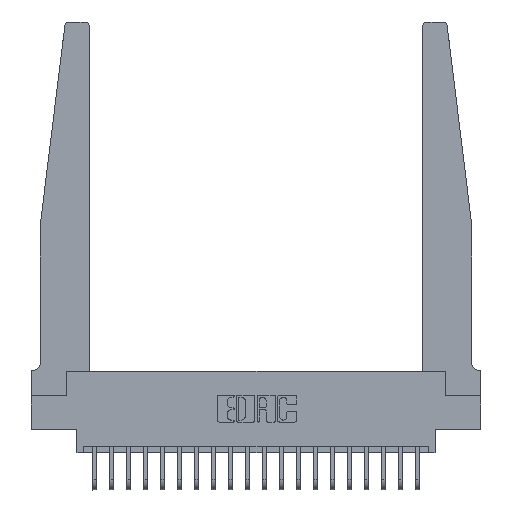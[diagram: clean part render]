
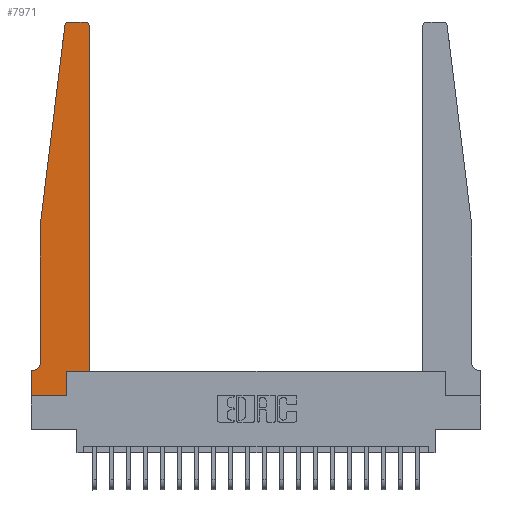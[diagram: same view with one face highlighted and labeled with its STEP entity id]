
A CAD part, top view. The second image highlights one B-rep face of the part: STEP entity #7971.
In plain terms, the highlighted planar face has unit normal (0, 0, 1).
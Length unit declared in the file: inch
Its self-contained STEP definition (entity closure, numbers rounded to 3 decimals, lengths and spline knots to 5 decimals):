
#485 = CARTESIAN_POINT ( 'NONE',  ( 0.015, 0.2375, 0.37 ) ) ;
#555 = VECTOR ( 'NONE', #1249, 39.37008 ) ;
#657 = DIRECTION ( 'NONE',  ( 1., 0., 0. ) ) ;
#1044 = CARTESIAN_POINT ( 'NONE',  ( 0.065, 1.25, 0.37 ) ) ;
#1048 = ORIENTED_EDGE ( 'NONE', *, *, #9518, .T. ) ;
#1143 = DIRECTION ( 'NONE',  ( 1., 0., 0. ) ) ;
#1249 = DIRECTION ( 'NONE',  ( 0., -1., 0. ) ) ;
#1559 = CIRCLE ( 'NONE', #14652, 0.03 ) ;
#1574 = CARTESIAN_POINT ( 'NONE',  ( 0.25, 2.75, 0.37 ) ) ;
#1659 = EDGE_CURVE ( 'NONE', #12723, #5210, #11822, .T. ) ;
#1767 = DIRECTION ( 'NONE',  ( 1., 0., 0. ) ) ;
#1916 = LINE ( 'NONE', #14757, #15223 ) ;
#2643 = ORIENTED_EDGE ( 'NONE', *, *, #12371, .T. ) ;
#2938 = DIRECTION ( 'NONE',  ( 0., 1., 0. ) ) ;
#3005 = CARTESIAN_POINT ( 'NONE',  ( 0., 0.1875, 0.37 ) ) ;
#3436 = ORIENTED_EDGE ( 'NONE', *, *, #12377, .T. ) ;
#3744 = DIRECTION ( 'NONE',  ( -1., 0., 0. ) ) ;
#4289 = VERTEX_POINT ( 'NONE', #7730 ) ;
#4322 = EDGE_CURVE ( 'NONE', #10886, #17482, #1916, .T. ) ;
#4595 = ORIENTED_EDGE ( 'NONE', *, *, #11111, .T. ) ;
#4912 = EDGE_CURVE ( 'NONE', #7193, #10886, #7055, .T. ) ;
#4939 = CARTESIAN_POINT ( 'NONE',  ( 0.065, 1.25, 0.37 ) ) ;
#5179 = VERTEX_POINT ( 'NONE', #4939 ) ;
#5210 = VERTEX_POINT ( 'NONE', #9680 ) ;
#5253 = AXIS2_PLACEMENT_3D ( 'NONE', #9687, #16196, #1767 ) ;
#5894 = DIRECTION ( 'NONE',  ( -0.122, -0.992, 0. ) ) ;
#6666 = ORIENTED_EDGE ( 'NONE', *, *, #4322, .T. ) ;
#7055 = LINE ( 'NONE', #13475, #9203 ) ;
#7065 = EDGE_LOOP ( 'NONE', ( #2643, #1048, #4595, #18231, #11783, #8671, #16813, #6666, #3436, #19146, #17581, #16800 ) ) ;
#7193 = VERTEX_POINT ( 'NONE', #3005 ) ;
#7730 = CARTESIAN_POINT ( 'NONE',  ( 0.24675, 2.72367, 0.37 ) ) ;
#7766 = CARTESIAN_POINT ( 'NONE',  ( 0.2605, 0.18, 0.37 ) ) ;
#7785 = FACE_OUTER_BOUND ( 'NONE', #7065, .T. ) ;
#7890 = LINE ( 'NONE', #1574, #15071 ) ;
#7891 = PLANE ( 'NONE',  #5253 ) ;
#7971 = ADVANCED_FACE ( 'NONE', ( #7785 ), #7891, .T. ) ;
#8057 = AXIS2_PLACEMENT_3D ( 'NONE', #485, #19723, #3744 ) ;
#8364 = CARTESIAN_POINT ( 'NONE',  ( 0.015, 0.1875, 0.37 ) ) ;
#8671 = ORIENTED_EDGE ( 'NONE', *, *, #13625, .T. ) ;
#8812 = CARTESIAN_POINT ( 'NONE',  ( 0.395, 2.75, 0.37 ) ) ;
#8916 = EDGE_CURVE ( 'NONE', #5210, #16633, #20361, .T. ) ;
#9148 = CARTESIAN_POINT ( 'NONE',  ( 0.27653, 2.72, 0.37 ) ) ;
#9203 = VECTOR ( 'NONE', #19871, 39.37008 ) ;
#9220 = CARTESIAN_POINT ( 'NONE',  ( 0.395, 2.72, 0.37 ) ) ;
#9425 = EDGE_CURVE ( 'NONE', #5179, #15299, #15664, .T. ) ;
#9518 = EDGE_CURVE ( 'NONE', #15981, #4289, #1559, .T. ) ;
#9571 = VERTEX_POINT ( 'NONE', #7766 ) ;
#9680 = CARTESIAN_POINT ( 'NONE',  ( 0.425, 2.72, 0.37 ) ) ;
#9687 = CARTESIAN_POINT ( 'NONE',  ( 0., 0.1875, 0.37 ) ) ;
#10753 = VECTOR ( 'NONE', #15056, 39.37008 ) ;
#10886 = VERTEX_POINT ( 'NONE', #17176 ) ;
#11013 = DIRECTION ( 'NONE',  ( 1., 0., 0. ) ) ;
#11061 = LINE ( 'NONE', #14408, #14752 ) ;
#11111 = EDGE_CURVE ( 'NONE', #4289, #5179, #12627, .T. ) ;
#11156 = CARTESIAN_POINT ( 'NONE',  ( 0.2605, 0.18, 0.37 ) ) ;
#11783 = ORIENTED_EDGE ( 'NONE', *, *, #14141, .T. ) ;
#11822 = LINE ( 'NONE', #15074, #17311 ) ;
#12371 = EDGE_CURVE ( 'NONE', #16633, #15981, #7890, .T. ) ;
#12377 = EDGE_CURVE ( 'NONE', #17482, #9571, #15586, .T. ) ;
#12627 = LINE ( 'NONE', #17154, #14053 ) ;
#12723 = VERTEX_POINT ( 'NONE', #15556 ) ;
#12733 = DIRECTION ( 'NONE',  ( -1., 0., 0. ) ) ;
#13258 = EDGE_CURVE ( 'NONE', #9571, #12723, #19674, .T. ) ;
#13302 = AXIS2_PLACEMENT_3D ( 'NONE', #9220, #15635, #11013 ) ;
#13475 = CARTESIAN_POINT ( 'NONE',  ( 0., 0., 0.37 ) ) ;
#13625 = EDGE_CURVE ( 'NONE', #18803, #7193, #11061, .T. ) ;
#14053 = VECTOR ( 'NONE', #5894, 39.37008 ) ;
#14141 = EDGE_CURVE ( 'NONE', #15299, #18803, #15117, .T. ) ;
#14408 = CARTESIAN_POINT ( 'NONE',  ( 0.065, 0.1875, 0.37 ) ) ;
#14652 = AXIS2_PLACEMENT_3D ( 'NONE', #9148, #15562, #1143 ) ;
#14722 = VECTOR ( 'NONE', #2938, 39.37008 ) ;
#14752 = VECTOR ( 'NONE', #20514, 39.37008 ) ;
#14757 = CARTESIAN_POINT ( 'NONE',  ( 0., 0., 0.37 ) ) ;
#15056 = DIRECTION ( 'NONE',  ( 1., 0., 0. ) ) ;
#15071 = VECTOR ( 'NONE', #12733, 39.37008 ) ;
#15074 = CARTESIAN_POINT ( 'NONE',  ( 0.425, 0.18, 0.37 ) ) ;
#15117 = CIRCLE ( 'NONE', #8057, 0.05 ) ;
#15223 = VECTOR ( 'NONE', #657, 39.37008 ) ;
#15299 = VERTEX_POINT ( 'NONE', #19913 ) ;
#15556 = CARTESIAN_POINT ( 'NONE',  ( 0.425, 0.18, 0.37 ) ) ;
#15562 = DIRECTION ( 'NONE',  ( 0., 0., 1. ) ) ;
#15586 = LINE ( 'NONE', #11156, #14722 ) ;
#15635 = DIRECTION ( 'NONE',  ( 0., 0., 1. ) ) ;
#15664 = LINE ( 'NONE', #1044, #555 ) ;
#15981 = VERTEX_POINT ( 'NONE', #16110 ) ;
#16110 = CARTESIAN_POINT ( 'NONE',  ( 0.27653, 2.75, 0.37 ) ) ;
#16196 = DIRECTION ( 'NONE',  ( 0., 0., 1. ) ) ;
#16633 = VERTEX_POINT ( 'NONE', #8812 ) ;
#16652 = DIRECTION ( 'NONE',  ( 0., 1., 0. ) ) ;
#16800 = ORIENTED_EDGE ( 'NONE', *, *, #8916, .T. ) ;
#16813 = ORIENTED_EDGE ( 'NONE', *, *, #4912, .T. ) ;
#17154 = CARTESIAN_POINT ( 'NONE',  ( 0.065, 1.25, 0.37 ) ) ;
#17176 = CARTESIAN_POINT ( 'NONE',  ( 0., 0., 0.37 ) ) ;
#17311 = VECTOR ( 'NONE', #16652, 39.37008 ) ;
#17482 = VERTEX_POINT ( 'NONE', #18609 ) ;
#17581 = ORIENTED_EDGE ( 'NONE', *, *, #1659, .T. ) ;
#17892 = CARTESIAN_POINT ( 'NONE',  ( 0.425, 0.18, 0.37 ) ) ;
#18231 = ORIENTED_EDGE ( 'NONE', *, *, #9425, .T. ) ;
#18609 = CARTESIAN_POINT ( 'NONE',  ( 0.2605, 0., 0.37 ) ) ;
#18803 = VERTEX_POINT ( 'NONE', #8364 ) ;
#19146 = ORIENTED_EDGE ( 'NONE', *, *, #13258, .T. ) ;
#19674 = LINE ( 'NONE', #17892, #10753 ) ;
#19723 = DIRECTION ( 'NONE',  ( 0., 0., -1. ) ) ;
#19871 = DIRECTION ( 'NONE',  ( 0., -1., 0. ) ) ;
#19913 = CARTESIAN_POINT ( 'NONE',  ( 0.065, 0.2375, 0.37 ) ) ;
#20361 = CIRCLE ( 'NONE', #13302, 0.03 ) ;
#20514 = DIRECTION ( 'NONE',  ( -1., 0., 0. ) ) ;
